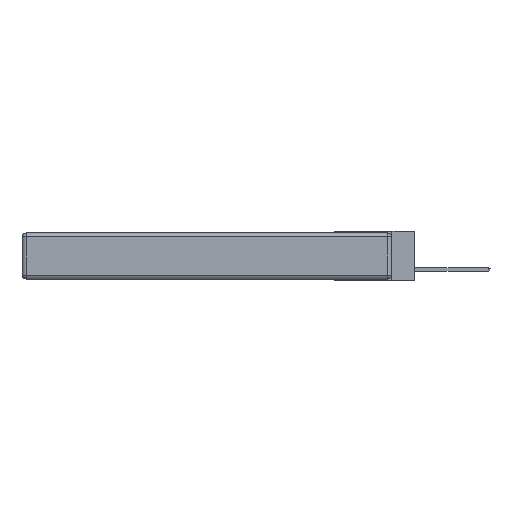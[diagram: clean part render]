
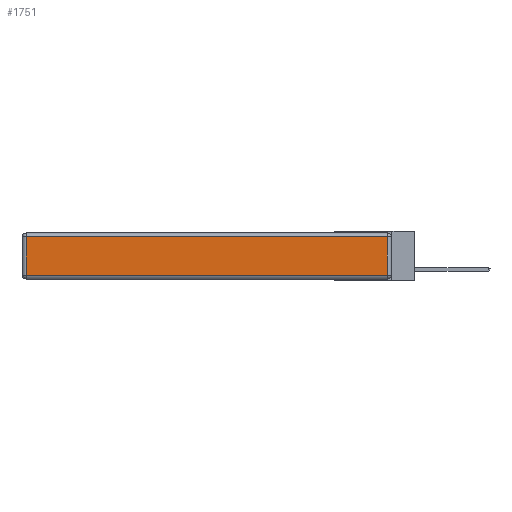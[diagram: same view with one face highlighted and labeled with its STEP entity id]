
A CAD part, left-side view. The second image highlights one B-rep face of the part: STEP entity #1751.
In plain terms, the highlighted planar face has unit normal (-1, 0, 0).
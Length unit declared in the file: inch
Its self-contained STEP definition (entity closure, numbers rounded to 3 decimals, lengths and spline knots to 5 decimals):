
#356 = ORIENTED_EDGE ( 'NONE', *, *, #4507, .T. ) ;
#771 = VERTEX_POINT ( 'NONE', #12014 ) ;
#994 = VERTEX_POINT ( 'NONE', #27378 ) ;
#1044 = CARTESIAN_POINT ( 'NONE',  ( 0., 2.75, -0.03 ) ) ;
#1099 = VERTEX_POINT ( 'NONE', #2856 ) ;
#1751 = ADVANCED_FACE ( 'NONE', ( #25155 ), #9241, .T. ) ;
#2856 = CARTESIAN_POINT ( 'NONE',  ( 0., 0.03, -0.313 ) ) ;
#3213 = ORIENTED_EDGE ( 'NONE', *, *, #22457, .T. ) ;
#4507 = EDGE_CURVE ( 'NONE', #14265, #1099, #11477, .T. ) ;
#5202 = LINE ( 'NONE', #1044, #14384 ) ;
#5214 = EDGE_CURVE ( 'NONE', #1099, #771, #10795, .T. ) ;
#6415 = DIRECTION ( 'NONE',  ( 0., -1., 0. ) ) ;
#8681 = DIRECTION ( 'NONE',  ( 0., 0., 1. ) ) ;
#9241 = PLANE ( 'NONE',  #16951 ) ;
#9449 = CARTESIAN_POINT ( 'NONE',  ( 0., 2.72, -0.343 ) ) ;
#10109 = VECTOR ( 'NONE', #8681, 39.37008 ) ;
#10383 = LINE ( 'NONE', #9449, #23237 ) ;
#10795 = LINE ( 'NONE', #18915, #10109 ) ;
#11477 = LINE ( 'NONE', #21523, #18935 ) ;
#11926 = DIRECTION ( 'NONE',  ( 0., 1., 0. ) ) ;
#12014 = CARTESIAN_POINT ( 'NONE',  ( 0., 0.03, -0.03 ) ) ;
#12292 = ORIENTED_EDGE ( 'NONE', *, *, #5214, .T. ) ;
#14184 = DIRECTION ( 'NONE',  ( 0., 0., -1. ) ) ;
#14265 = VERTEX_POINT ( 'NONE', #15025 ) ;
#14384 = VECTOR ( 'NONE', #11926, 39.37008 ) ;
#15025 = CARTESIAN_POINT ( 'NONE',  ( 0., 2.72, -0.313 ) ) ;
#16365 = EDGE_CURVE ( 'NONE', #994, #14265, #10383, .T. ) ;
#16951 = AXIS2_PLACEMENT_3D ( 'NONE', #24189, #22963, #18598 ) ;
#18598 = DIRECTION ( 'NONE',  ( 0., 0., 1. ) ) ;
#18915 = CARTESIAN_POINT ( 'NONE',  ( 0., 0.03, -0.343 ) ) ;
#18935 = VECTOR ( 'NONE', #6415, 39.37008 ) ;
#21523 = CARTESIAN_POINT ( 'NONE',  ( 0., 0., -0.313 ) ) ;
#22457 = EDGE_CURVE ( 'NONE', #771, #994, #5202, .T. ) ;
#22963 = DIRECTION ( 'NONE',  ( -1., 0., 0. ) ) ;
#23237 = VECTOR ( 'NONE', #14184, 39.37008 ) ;
#24189 = CARTESIAN_POINT ( 'NONE',  ( 0., 0., -0.343 ) ) ;
#24655 = ORIENTED_EDGE ( 'NONE', *, *, #16365, .T. ) ;
#25155 = FACE_OUTER_BOUND ( 'NONE', #27647, .T. ) ;
#27378 = CARTESIAN_POINT ( 'NONE',  ( 0., 2.72, -0.03 ) ) ;
#27647 = EDGE_LOOP ( 'NONE', ( #356, #12292, #3213, #24655 ) ) ;
